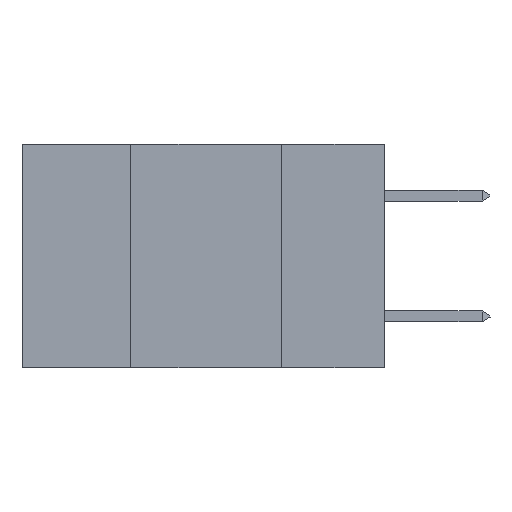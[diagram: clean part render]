
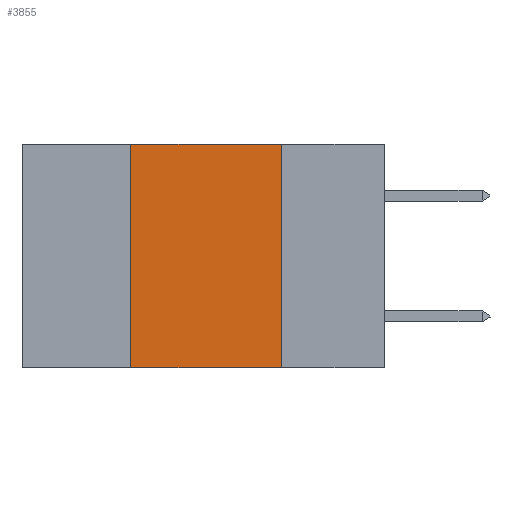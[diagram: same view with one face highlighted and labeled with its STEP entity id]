
A CAD part, left-side view. The second image highlights one B-rep face of the part: STEP entity #3855.
In plain terms, the highlighted planar face has unit normal (-1, 0, 0).
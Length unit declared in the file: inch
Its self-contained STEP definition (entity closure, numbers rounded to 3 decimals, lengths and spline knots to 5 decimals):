
#330 = DIRECTION ( 'NONE',  ( 0., -1., 0. ) ) ;
#360 = CARTESIAN_POINT ( 'NONE',  ( 0., 0.17, -0.37 ) ) ;
#660 = VECTOR ( 'NONE', #16185, 39.37008 ) ;
#832 = CARTESIAN_POINT ( 'NONE',  ( 0., 0.42, -0.37 ) ) ;
#1135 = CARTESIAN_POINT ( 'NONE',  ( 0., 0.42, 0. ) ) ;
#1440 = VERTEX_POINT ( 'NONE', #832 ) ;
#1587 = CARTESIAN_POINT ( 'NONE',  ( 0., 0.6, 0. ) ) ;
#2371 = VERTEX_POINT ( 'NONE', #1135 ) ;
#2706 = DIRECTION ( 'NONE',  ( 0., 0., -1. ) ) ;
#2815 = ORIENTED_EDGE ( 'NONE', *, *, #11738, .F. ) ;
#2987 = VERTEX_POINT ( 'NONE', #14123 ) ;
#3855 = ADVANCED_FACE ( 'NONE', ( #9293 ), #7739, .F. ) ;
#3916 = ORIENTED_EDGE ( 'NONE', *, *, #4315, .T. ) ;
#4075 = DIRECTION ( 'NONE',  ( 1., 0., 0. ) ) ;
#4315 = EDGE_CURVE ( 'NONE', #1440, #5075, #7291, .T. ) ;
#4887 = VECTOR ( 'NONE', #2706, 39.37008 ) ;
#5075 = VERTEX_POINT ( 'NONE', #360 ) ;
#5320 = VECTOR ( 'NONE', #13185, 39.37008 ) ;
#5972 = EDGE_CURVE ( 'NONE', #1440, #2371, #6703, .T. ) ;
#6703 = LINE ( 'NONE', #14290, #5320 ) ;
#7145 = LINE ( 'NONE', #14032, #9844 ) ;
#7291 = LINE ( 'NONE', #9883, #660 ) ;
#7300 = ORIENTED_EDGE ( 'NONE', *, *, #5972, .F. ) ;
#7739 = PLANE ( 'NONE',  #14207 ) ;
#7995 = DIRECTION ( 'NONE',  ( 0., 0., -1. ) ) ;
#8557 = EDGE_CURVE ( 'NONE', #2987, #5075, #15854, .T. ) ;
#9293 = FACE_OUTER_BOUND ( 'NONE', #9737, .T. ) ;
#9737 = EDGE_LOOP ( 'NONE', ( #12877, #2815, #7300, #3916 ) ) ;
#9844 = VECTOR ( 'NONE', #330, 39.37008 ) ;
#9883 = CARTESIAN_POINT ( 'NONE',  ( 0., 0.6, -0.37 ) ) ;
#11738 = EDGE_CURVE ( 'NONE', #2371, #2987, #7145, .T. ) ;
#12877 = ORIENTED_EDGE ( 'NONE', *, *, #8557, .F. ) ;
#13185 = DIRECTION ( 'NONE',  ( 0., 0., 1. ) ) ;
#14032 = CARTESIAN_POINT ( 'NONE',  ( 0., 0.6, 0. ) ) ;
#14084 = CARTESIAN_POINT ( 'NONE',  ( 0., 0.17, 0. ) ) ;
#14123 = CARTESIAN_POINT ( 'NONE',  ( 0., 0.17, 0. ) ) ;
#14207 = AXIS2_PLACEMENT_3D ( 'NONE', #1587, #4075, #7995 ) ;
#14290 = CARTESIAN_POINT ( 'NONE',  ( 0., 0.42, 0. ) ) ;
#15854 = LINE ( 'NONE', #14084, #4887 ) ;
#16185 = DIRECTION ( 'NONE',  ( 0., -1., 0. ) ) ;
